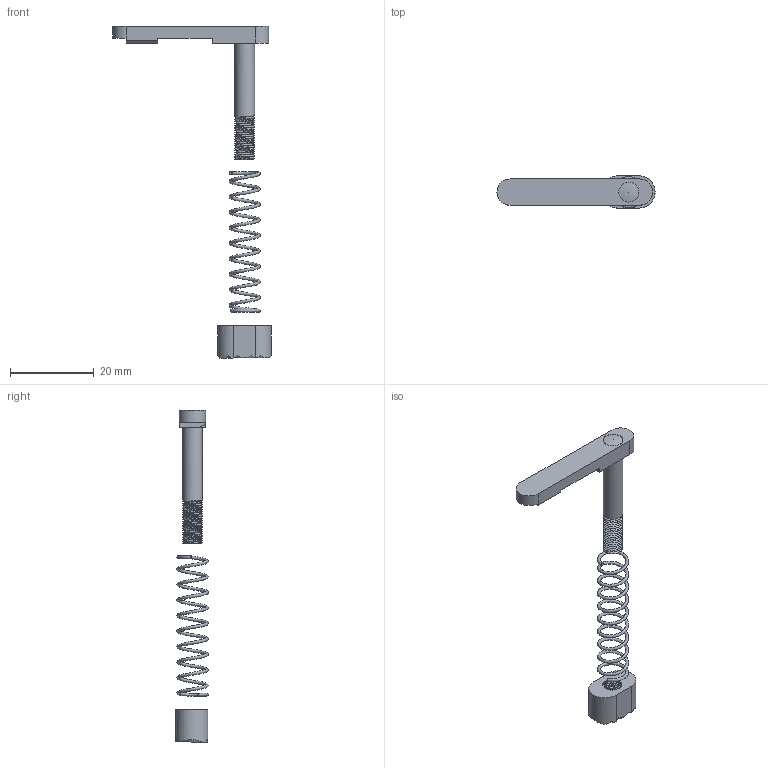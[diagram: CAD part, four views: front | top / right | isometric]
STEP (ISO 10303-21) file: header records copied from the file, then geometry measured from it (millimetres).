
FILE_DESCRIPTION(/* description */ (''),/* implementation_level */ '2;1');
FILE_NAME(/* name */ 'mag release.stp',/* time_stamp */ '2014-08-27T22:01:57-04:00',/* author */ ('Workstation'),/* organization */ (''),/* preprocessor_version */ 'ST-DEVELOPER v15.2',/* originating_system */ 'Autodesk Inventor 2014',/* authorisation */ '');
FILE_SCHEMA (('AUTOMOTIVE_DESIGN { 1 0 10303 214 3 1 1 }'));
Length unit declared in the file: inch
Products named in the file (5): Solid5; Solid6; Solid4; Solid2; mag release
Bounding box: 37.72 x 7.71 x 79.17 mm (x, y, z)
Volume: 1851 mm3; surface area: 2498.7 mm2
Topology: 4 solids, 4 shells, 50 faces, 126 edges, 84 vertices
Faces by surface type: plane 25, cone 12, cylinder 7, bspline 6
Full cylindrical faces by diameter (mm): 4.75 x2
Entity records: 13241 total; most frequent: CARTESIAN_POINT 12019, ORIENTED_EDGE 236, DIRECTION 228, EDGE_CURVE 118, AXIS2_PLACEMENT_3D 93, VERTEX_POINT 82, EDGE_LOOP 60, ADVANCED_FACE 50
